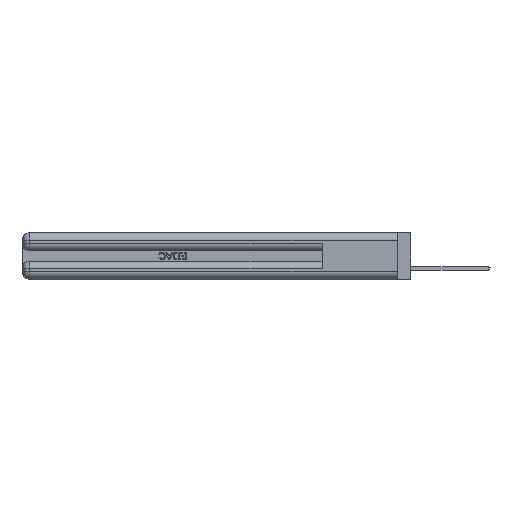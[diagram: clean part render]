
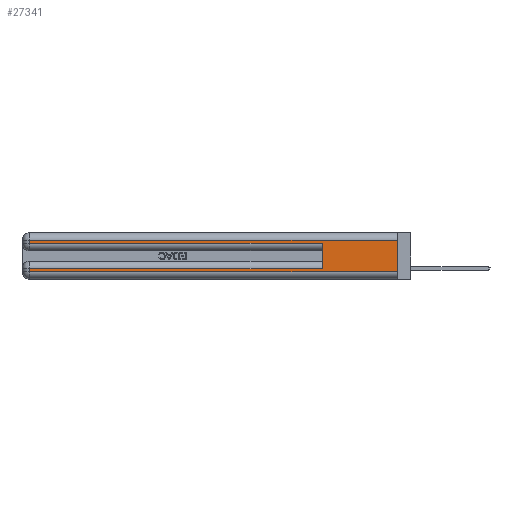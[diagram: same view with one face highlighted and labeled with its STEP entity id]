
A CAD part, left-side view. The second image highlights one B-rep face of the part: STEP entity #27341.
In plain terms, the highlighted planar face has unit normal (-1, 0, 0).
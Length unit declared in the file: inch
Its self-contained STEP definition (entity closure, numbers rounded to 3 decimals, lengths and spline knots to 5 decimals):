
#637 = DIRECTION ( 'NONE',  ( 0., 0., 1. ) ) ;
#988 = CARTESIAN_POINT ( 'NONE',  ( 0., 0.6, 0.145 ) ) ;
#1493 = CARTESIAN_POINT ( 'NONE',  ( 0., 0.6, 0.085 ) ) ;
#2153 = EDGE_CURVE ( 'NONE', #45669, #12695, #45814, .T. ) ;
#2362 = EDGE_CURVE ( 'NONE', #32511, #26154, #6754, .T. ) ;
#4392 = DIRECTION ( 'NONE',  ( 0., 1., 0. ) ) ;
#4962 = ORIENTED_EDGE ( 'NONE', *, *, #26629, .T. ) ;
#5472 = EDGE_CURVE ( 'NONE', #39398, #44836, #38436, .T. ) ;
#6754 = LINE ( 'NONE', #15487, #48215 ) ;
#7798 = CARTESIAN_POINT ( 'NONE',  ( 0., 0., 0.06 ) ) ;
#8178 = CARTESIAN_POINT ( 'NONE',  ( 0., 0., 0.37 ) ) ;
#10337 = VERTEX_POINT ( 'NONE', #1493 ) ;
#11107 = CARTESIAN_POINT ( 'NONE',  ( 0., 2.94, 0.31 ) ) ;
#12695 = VERTEX_POINT ( 'NONE', #11107 ) ;
#12901 = VECTOR ( 'NONE', #35852, 39.37008 ) ;
#12977 = ORIENTED_EDGE ( 'NONE', *, *, #5472, .T. ) ;
#15487 = CARTESIAN_POINT ( 'NONE',  ( 0., 0., 0.06 ) ) ;
#15596 = AXIS2_PLACEMENT_3D ( 'NONE', #41336, #45256, #22107 ) ;
#17308 = VECTOR ( 'NONE', #4392, 39.37008 ) ;
#18480 = FACE_OUTER_BOUND ( 'NONE', #28439, .T. ) ;
#19198 = CARTESIAN_POINT ( 'NONE',  ( 0., 0., 0.31 ) ) ;
#21986 = CARTESIAN_POINT ( 'NONE',  ( 0., 2.94, 0.37 ) ) ;
#22107 = DIRECTION ( 'NONE',  ( 0., 0., -1. ) ) ;
#22192 = LINE ( 'NONE', #30312, #17308 ) ;
#24023 = ORIENTED_EDGE ( 'NONE', *, *, #29379, .T. ) ;
#24763 = CARTESIAN_POINT ( 'NONE',  ( 0., 2.94, 0.085 ) ) ;
#26154 = VERTEX_POINT ( 'NONE', #7798 ) ;
#26629 = EDGE_CURVE ( 'NONE', #10337, #29261, #22192, .T. ) ;
#27115 = DIRECTION ( 'NONE',  ( 0., -1., 0. ) ) ;
#27341 = ADVANCED_FACE ( 'NONE', ( #18480 ), #49690, .F. ) ;
#28409 = ORIENTED_EDGE ( 'NONE', *, *, #50453, .F. ) ;
#28439 = EDGE_LOOP ( 'NONE', ( #49600, #32943, #24023, #12977, #28409, #4962, #41027, #49076 ) ) ;
#29261 = VERTEX_POINT ( 'NONE', #24763 ) ;
#29379 = EDGE_CURVE ( 'NONE', #12695, #39398, #29623, .T. ) ;
#29623 = LINE ( 'NONE', #21986, #42975 ) ;
#30312 = CARTESIAN_POINT ( 'NONE',  ( 0., 0., 0.085 ) ) ;
#30711 = CARTESIAN_POINT ( 'NONE',  ( 0., 2.94, 0.06 ) ) ;
#32511 = VERTEX_POINT ( 'NONE', #30711 ) ;
#32943 = ORIENTED_EDGE ( 'NONE', *, *, #2153, .T. ) ;
#34490 = LINE ( 'NONE', #988, #38118 ) ;
#34768 = EDGE_CURVE ( 'NONE', #45669, #26154, #45275, .T. ) ;
#35276 = DIRECTION ( 'NONE',  ( 0., -1., 0. ) ) ;
#35852 = DIRECTION ( 'NONE',  ( 0., 1., 0. ) ) ;
#37862 = EDGE_CURVE ( 'NONE', #29261, #32511, #45286, .T. ) ;
#38118 = VECTOR ( 'NONE', #637, 39.37008 ) ;
#38436 = LINE ( 'NONE', #41878, #42065 ) ;
#39398 = VERTEX_POINT ( 'NONE', #43526 ) ;
#40233 = CARTESIAN_POINT ( 'NONE',  ( 0., 0.6, 0.285 ) ) ;
#40392 = VECTOR ( 'NONE', #47379, 39.37008 ) ;
#41027 = ORIENTED_EDGE ( 'NONE', *, *, #37862, .T. ) ;
#41336 = CARTESIAN_POINT ( 'NONE',  ( 0., 0., 0.37 ) ) ;
#41878 = CARTESIAN_POINT ( 'NONE',  ( 0., 0., 0.285 ) ) ;
#42065 = VECTOR ( 'NONE', #27115, 39.37008 ) ;
#42975 = VECTOR ( 'NONE', #45130, 39.37008 ) ;
#43526 = CARTESIAN_POINT ( 'NONE',  ( 0., 2.94, 0.285 ) ) ;
#44066 = VECTOR ( 'NONE', #49915, 39.37008 ) ;
#44836 = VERTEX_POINT ( 'NONE', #40233 ) ;
#45130 = DIRECTION ( 'NONE',  ( 0., 0., -1. ) ) ;
#45256 = DIRECTION ( 'NONE',  ( 1., 0., 0. ) ) ;
#45275 = LINE ( 'NONE', #8178, #40392 ) ;
#45286 = LINE ( 'NONE', #45981, #44066 ) ;
#45669 = VERTEX_POINT ( 'NONE', #19198 ) ;
#45814 = LINE ( 'NONE', #47732, #12901 ) ;
#45981 = CARTESIAN_POINT ( 'NONE',  ( 0., 2.94, 0.37 ) ) ;
#47379 = DIRECTION ( 'NONE',  ( 0., 0., -1. ) ) ;
#47732 = CARTESIAN_POINT ( 'NONE',  ( 0., 0., 0.31 ) ) ;
#48215 = VECTOR ( 'NONE', #35276, 39.37008 ) ;
#49076 = ORIENTED_EDGE ( 'NONE', *, *, #2362, .T. ) ;
#49600 = ORIENTED_EDGE ( 'NONE', *, *, #34768, .F. ) ;
#49690 = PLANE ( 'NONE',  #15596 ) ;
#49915 = DIRECTION ( 'NONE',  ( 0., 0., -1. ) ) ;
#50453 = EDGE_CURVE ( 'NONE', #10337, #44836, #34490, .T. ) ;
